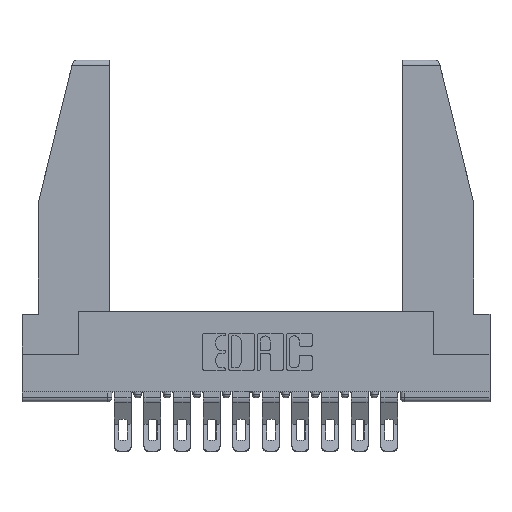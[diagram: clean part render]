
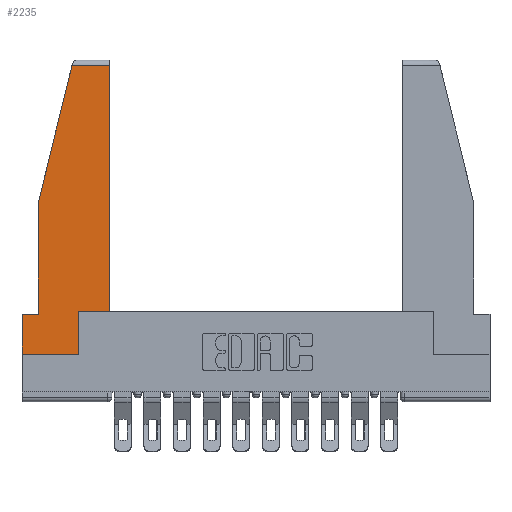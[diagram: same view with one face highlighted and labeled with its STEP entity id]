
A CAD part, top view. The second image highlights one B-rep face of the part: STEP entity #2235.
In plain terms, the highlighted planar face has unit normal (0, 0, 1).
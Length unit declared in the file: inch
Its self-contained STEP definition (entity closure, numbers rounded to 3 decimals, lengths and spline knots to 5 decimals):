
#117 = VERTEX_POINT ( 'NONE', #13250 ) ;
#624 = EDGE_CURVE ( 'NONE', #9828, #12963, #10403, .T. ) ;
#679 = DIRECTION ( 'NONE',  ( 1., 0., 0. ) ) ;
#1008 = CARTESIAN_POINT ( 'NONE',  ( 0., 0., 0. ) ) ;
#1090 = VERTEX_POINT ( 'NONE', #1008 ) ;
#1235 = EDGE_CURVE ( 'NONE', #14320, #1090, #3950, .T. ) ;
#1249 = EDGE_CURVE ( 'NONE', #12745, #1763, #13717, .T. ) ;
#1666 = ORIENTED_EDGE ( 'NONE', *, *, #1249, .T. ) ;
#1749 = ORIENTED_EDGE ( 'NONE', *, *, #624, .T. ) ;
#1763 = VERTEX_POINT ( 'NONE', #9523 ) ;
#1860 = VECTOR ( 'NONE', #13793, 39.37008 ) ;
#1961 = ORIENTED_EDGE ( 'NONE', *, *, #15530, .T. ) ;
#2133 = CARTESIAN_POINT ( 'NONE',  ( 0.086, 0.8, 0. ) ) ;
#2235 = ADVANCED_FACE ( 'NONE', ( #5194 ), #10093, .T. ) ;
#2578 = CARTESIAN_POINT ( 'NONE',  ( 0., 1.52, 0. ) ) ;
#2954 = VECTOR ( 'NONE', #3142, 39.37008 ) ;
#3074 = ORIENTED_EDGE ( 'NONE', *, *, #15804, .T. ) ;
#3142 = DIRECTION ( 'NONE',  ( 0., 1., 0. ) ) ;
#3538 = LINE ( 'NONE', #7490, #12054 ) ;
#3950 = LINE ( 'NONE', #5230, #1860 ) ;
#4302 = VERTEX_POINT ( 'NONE', #8676 ) ;
#4523 = ORIENTED_EDGE ( 'NONE', *, *, #10745, .T. ) ;
#5194 = FACE_OUTER_BOUND ( 'NONE', #8244, .T. ) ;
#5230 = CARTESIAN_POINT ( 'NONE',  ( 0., 0.21, 0. ) ) ;
#5284 = CARTESIAN_POINT ( 'NONE',  ( 0.297, 0., 0. ) ) ;
#5950 = VECTOR ( 'NONE', #10129, 39.37008 ) ;
#6187 = CARTESIAN_POINT ( 'NONE',  ( 0., 0., 0. ) ) ;
#6961 = CARTESIAN_POINT ( 'NONE',  ( 0.086, 0.21, 0. ) ) ;
#7490 = CARTESIAN_POINT ( 'NONE',  ( 0., 0.21, 0. ) ) ;
#7583 = ORIENTED_EDGE ( 'NONE', *, *, #13294, .T. ) ;
#7626 = LINE ( 'NONE', #5284, #9063 ) ;
#7632 = DIRECTION ( 'NONE',  ( 1., 0., 0. ) ) ;
#7732 = CARTESIAN_POINT ( 'NONE',  ( 0.297, 0.223, 0. ) ) ;
#7739 = CARTESIAN_POINT ( 'NONE',  ( 0.461, 0.223, 0. ) ) ;
#7756 = VERTEX_POINT ( 'NONE', #6961 ) ;
#7984 = LINE ( 'NONE', #7739, #2954 ) ;
#8244 = EDGE_LOOP ( 'NONE', ( #3074, #1666, #10579, #1961, #12848, #15775, #7583, #4523, #1749 ) ) ;
#8275 = AXIS2_PLACEMENT_3D ( 'NONE', #14969, #8905, #679 ) ;
#8494 = LINE ( 'NONE', #2133, #12668 ) ;
#8676 = CARTESIAN_POINT ( 'NONE',  ( 0.297, 0., 0. ) ) ;
#8722 = CARTESIAN_POINT ( 'NONE',  ( 0.461, 1.52, 0. ) ) ;
#8820 = EDGE_CURVE ( 'NONE', #7756, #14320, #3538, .T. ) ;
#8905 = DIRECTION ( 'NONE',  ( 0., 0., 1. ) ) ;
#9057 = DIRECTION ( 'NONE',  ( 1., 0., 0. ) ) ;
#9063 = VECTOR ( 'NONE', #14907, 39.37008 ) ;
#9092 = VECTOR ( 'NONE', #7632, 39.37008 ) ;
#9523 = CARTESIAN_POINT ( 'NONE',  ( 0.2636, 1.52, 0. ) ) ;
#9752 = DIRECTION ( 'NONE',  ( -1., 0., 0. ) ) ;
#9828 = VERTEX_POINT ( 'NONE', #7732 ) ;
#10093 = PLANE ( 'NONE',  #8275 ) ;
#10129 = DIRECTION ( 'NONE',  ( -1., 0., 0. ) ) ;
#10366 = CARTESIAN_POINT ( 'NONE',  ( 0.461, 0.223, 0. ) ) ;
#10387 = CARTESIAN_POINT ( 'NONE',  ( 0., 0.21, 0. ) ) ;
#10403 = LINE ( 'NONE', #12860, #11327 ) ;
#10492 = LINE ( 'NONE', #14002, #12177 ) ;
#10579 = ORIENTED_EDGE ( 'NONE', *, *, #15154, .T. ) ;
#10745 = EDGE_CURVE ( 'NONE', #4302, #9828, #7626, .T. ) ;
#11327 = VECTOR ( 'NONE', #9057, 39.37008 ) ;
#12054 = VECTOR ( 'NONE', #9752, 39.37008 ) ;
#12177 = VECTOR ( 'NONE', #14079, 39.37008 ) ;
#12668 = VECTOR ( 'NONE', #13339, 39.37008 ) ;
#12745 = VERTEX_POINT ( 'NONE', #8722 ) ;
#12848 = ORIENTED_EDGE ( 'NONE', *, *, #8820, .T. ) ;
#12860 = CARTESIAN_POINT ( 'NONE',  ( 0.297, 0.223, 0. ) ) ;
#12963 = VERTEX_POINT ( 'NONE', #10366 ) ;
#13250 = CARTESIAN_POINT ( 'NONE',  ( 0.086, 0.8, 0. ) ) ;
#13294 = EDGE_CURVE ( 'NONE', #1090, #4302, #14914, .T. ) ;
#13339 = DIRECTION ( 'NONE',  ( 0., -1., 0. ) ) ;
#13717 = LINE ( 'NONE', #2578, #5950 ) ;
#13793 = DIRECTION ( 'NONE',  ( 0., -1., 0. ) ) ;
#14002 = CARTESIAN_POINT ( 'NONE',  ( 0.271, 1.55, 0. ) ) ;
#14079 = DIRECTION ( 'NONE',  ( -0.239, -0.971, 0. ) ) ;
#14320 = VERTEX_POINT ( 'NONE', #10387 ) ;
#14907 = DIRECTION ( 'NONE',  ( 0., 1., 0. ) ) ;
#14914 = LINE ( 'NONE', #6187, #9092 ) ;
#14969 = CARTESIAN_POINT ( 'NONE',  ( 0., 0., 0. ) ) ;
#15154 = EDGE_CURVE ( 'NONE', #1763, #117, #10492, .T. ) ;
#15530 = EDGE_CURVE ( 'NONE', #117, #7756, #8494, .T. ) ;
#15775 = ORIENTED_EDGE ( 'NONE', *, *, #1235, .T. ) ;
#15804 = EDGE_CURVE ( 'NONE', #12963, #12745, #7984, .T. ) ;
